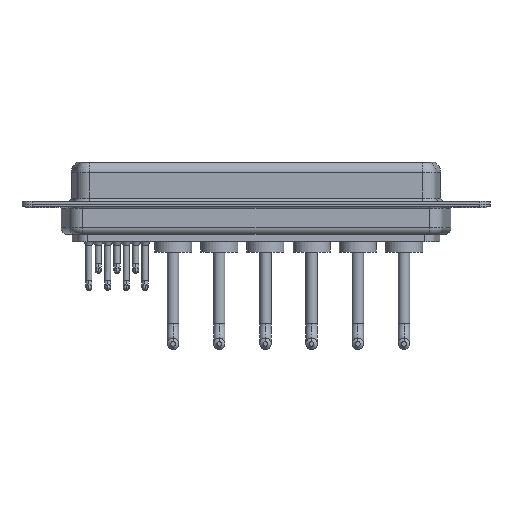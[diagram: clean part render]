
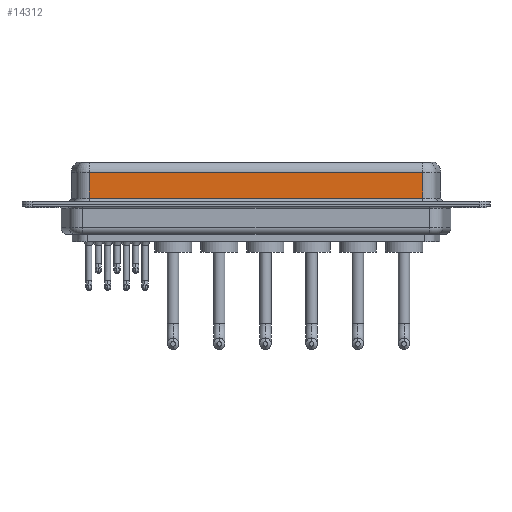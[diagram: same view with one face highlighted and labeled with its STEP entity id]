
A CAD part, front view. The second image highlights one B-rep face of the part: STEP entity #14312.
In plain terms, the highlighted planar face has unit normal (0, -1, 0).
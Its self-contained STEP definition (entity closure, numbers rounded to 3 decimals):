
#37 = VERTEX_POINT ( 'NONE', #1971 ) ;
#128 = VERTEX_POINT ( 'NONE', #8358 ) ;
#183 = VERTEX_POINT ( 'NONE', #4734 ) ;
#1014 = DIRECTION ( 'NONE',  ( 0., 1., 0. ) ) ;
#1695 = ORIENTED_EDGE ( 'NONE', *, *, #13515, .T. ) ;
#1837 = CARTESIAN_POINT ( 'NONE',  ( 7.038, -3.95, 6.4 ) ) ;
#1963 = AXIS2_PLACEMENT_3D ( 'NONE', #11606, #1014, #3794 ) ;
#1971 = CARTESIAN_POINT ( 'NONE',  ( 7.038, -3.95, 0.9 ) ) ;
#1975 = ORIENTED_EDGE ( 'NONE', *, *, #11391, .F. ) ;
#2475 = EDGE_CURVE ( 'NONE', #183, #13957, #12733, .T. ) ;
#2532 = PLANE ( 'NONE',  #1963 ) ;
#2607 = ORIENTED_EDGE ( 'NONE', *, *, #3473, .T. ) ;
#3257 = DIRECTION ( 'NONE',  ( 0., 0., -1. ) ) ;
#3473 = EDGE_CURVE ( 'NONE', #13957, #37, #9477, .T. ) ;
#3794 = DIRECTION ( 'NONE',  ( 0., 0., 1. ) ) ;
#3840 = VECTOR ( 'NONE', #12007, 1000. ) ;
#3982 = CARTESIAN_POINT ( 'NONE',  ( 56.462, -3.95, 4.65 ) ) ;
#4428 = LINE ( 'NONE', #14927, #9181 ) ;
#4734 = CARTESIAN_POINT ( 'NONE',  ( 56.462, -3.95, 4.65 ) ) ;
#5447 = LINE ( 'NONE', #8054, #3840 ) ;
#8054 = CARTESIAN_POINT ( 'NONE',  ( 56.462, -3.95, 0.9 ) ) ;
#8295 = DIRECTION ( 'NONE',  ( 0., 0., -1. ) ) ;
#8358 = CARTESIAN_POINT ( 'NONE',  ( 56.462, -3.95, 0.9 ) ) ;
#8405 = VECTOR ( 'NONE', #9107, 1000. ) ;
#9107 = DIRECTION ( 'NONE',  ( -1., 0., 0. ) ) ;
#9181 = VECTOR ( 'NONE', #8295, 1000. ) ;
#9477 = LINE ( 'NONE', #1837, #11537 ) ;
#9715 = ORIENTED_EDGE ( 'NONE', *, *, #2475, .T. ) ;
#10045 = EDGE_LOOP ( 'NONE', ( #1975, #9715, #2607, #1695 ) ) ;
#11391 = EDGE_CURVE ( 'NONE', #183, #128, #4428, .T. ) ;
#11537 = VECTOR ( 'NONE', #3257, 1000. ) ;
#11606 = CARTESIAN_POINT ( 'NONE',  ( 56.462, -3.95, 6.4 ) ) ;
#12007 = DIRECTION ( 'NONE',  ( 1., 0., 0. ) ) ;
#12733 = LINE ( 'NONE', #3982, #8405 ) ;
#13317 = CARTESIAN_POINT ( 'NONE',  ( 7.038, -3.95, 4.65 ) ) ;
#13515 = EDGE_CURVE ( 'NONE', #37, #128, #5447, .T. ) ;
#13778 = FACE_OUTER_BOUND ( 'NONE', #10045, .T. ) ;
#13957 = VERTEX_POINT ( 'NONE', #13317 ) ;
#14312 = ADVANCED_FACE ( 'NONE', ( #13778 ), #2532, .F. ) ;
#14927 = CARTESIAN_POINT ( 'NONE',  ( 56.462, -3.95, 6.4 ) ) ;
